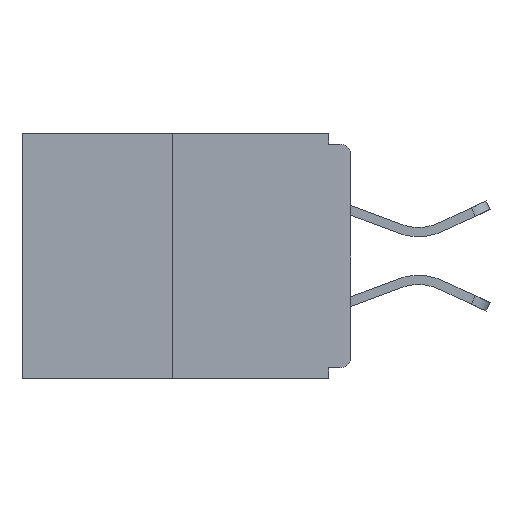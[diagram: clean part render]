
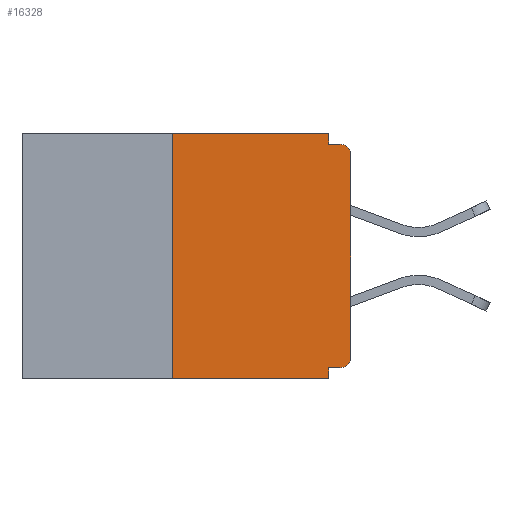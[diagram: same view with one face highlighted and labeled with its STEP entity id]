
A CAD part, left-side view. The second image highlights one B-rep face of the part: STEP entity #16328.
In plain terms, the highlighted planar face has unit normal (-1, 0, 0).
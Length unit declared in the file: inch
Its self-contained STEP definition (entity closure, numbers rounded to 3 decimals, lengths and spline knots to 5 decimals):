
#82 = VERTEX_POINT ( 'NONE', #6272 ) ;
#199 = CARTESIAN_POINT ( 'NONE',  ( 0., 0., -0.328 ) ) ;
#245 = CARTESIAN_POINT ( 'NONE',  ( 0., 0., -0.015 ) ) ;
#478 = VERTEX_POINT ( 'NONE', #7703 ) ;
#950 = ORIENTED_EDGE ( 'NONE', *, *, #20727, .T. ) ;
#986 = FACE_OUTER_BOUND ( 'NONE', #14619, .T. ) ;
#1017 = EDGE_CURVE ( 'NONE', #19914, #82, #13532, .T. ) ;
#1973 = CARTESIAN_POINT ( 'NONE',  ( 0., 0.031, 0. ) ) ;
#2096 = EDGE_CURVE ( 'NONE', #478, #8145, #9523, .T. ) ;
#2396 = CARTESIAN_POINT ( 'NONE',  ( 0., 0., 0. ) ) ;
#2826 = CARTESIAN_POINT ( 'NONE',  ( 0., 0.46, 0. ) ) ;
#3146 = VERTEX_POINT ( 'NONE', #3732 ) ;
#3207 = VECTOR ( 'NONE', #7239, 39.37008 ) ;
#3417 = VERTEX_POINT ( 'NONE', #3464 ) ;
#3464 = CARTESIAN_POINT ( 'NONE',  ( 0., 0.015, -0.328 ) ) ;
#3565 = LINE ( 'NONE', #245, #15094 ) ;
#3603 = VECTOR ( 'NONE', #21487, 39.37008 ) ;
#3732 = CARTESIAN_POINT ( 'NONE',  ( 0., 0.25, -0.343 ) ) ;
#4005 = VECTOR ( 'NONE', #13349, 39.37008 ) ;
#4217 = DIRECTION ( 'NONE',  ( 0., 0., -1. ) ) ;
#4445 = CARTESIAN_POINT ( 'NONE',  ( 0., 0.46, 0. ) ) ;
#4777 = VERTEX_POINT ( 'NONE', #11687 ) ;
#4943 = EDGE_CURVE ( 'NONE', #3417, #478, #10783, .T. ) ;
#5221 = ORIENTED_EDGE ( 'NONE', *, *, #20174, .T. ) ;
#5307 = CARTESIAN_POINT ( 'NONE',  ( 0., 0.25, 0. ) ) ;
#5667 = DIRECTION ( 'NONE',  ( 0., 0., -1. ) ) ;
#6024 = CIRCLE ( 'NONE', #18871, 0.015 ) ;
#6272 = CARTESIAN_POINT ( 'NONE',  ( 0., 0.031, -0.015 ) ) ;
#6292 = CARTESIAN_POINT ( 'NONE',  ( 0., 0.031, -0.343 ) ) ;
#6372 = EDGE_CURVE ( 'NONE', #3146, #19278, #20629, .T. ) ;
#6813 = EDGE_CURVE ( 'NONE', #3146, #8145, #17569, .T. ) ;
#6817 = CARTESIAN_POINT ( 'NONE',  ( 0., 0.25, 0. ) ) ;
#6891 = DIRECTION ( 'NONE',  ( 0., 0., 1. ) ) ;
#7239 = DIRECTION ( 'NONE',  ( 0., 0., 1. ) ) ;
#7465 = AXIS2_PLACEMENT_3D ( 'NONE', #8396, #17013, #11736 ) ;
#7703 = CARTESIAN_POINT ( 'NONE',  ( 0., 0.031, -0.328 ) ) ;
#8145 = VERTEX_POINT ( 'NONE', #12028 ) ;
#8396 = CARTESIAN_POINT ( 'NONE',  ( 0., 0.015, -0.03 ) ) ;
#8596 = DIRECTION ( 'NONE',  ( -1., 0., 0. ) ) ;
#8708 = CARTESIAN_POINT ( 'NONE',  ( 0., 0., -0.313 ) ) ;
#9095 = ORIENTED_EDGE ( 'NONE', *, *, #11487, .F. ) ;
#9523 = LINE ( 'NONE', #6292, #3603 ) ;
#10064 = VERTEX_POINT ( 'NONE', #8708 ) ;
#10783 = LINE ( 'NONE', #199, #12243 ) ;
#11331 = ORIENTED_EDGE ( 'NONE', *, *, #6813, .T. ) ;
#11487 = EDGE_CURVE ( 'NONE', #82, #12473, #3565, .T. ) ;
#11687 = CARTESIAN_POINT ( 'NONE',  ( 0., 0., -0.03 ) ) ;
#11736 = DIRECTION ( 'NONE',  ( 0., 0., -1. ) ) ;
#11744 = CARTESIAN_POINT ( 'NONE',  ( 0., 0.031, 0. ) ) ;
#12028 = CARTESIAN_POINT ( 'NONE',  ( 0., 0.031, -0.343 ) ) ;
#12156 = CARTESIAN_POINT ( 'NONE',  ( 0., 0.015, -0.313 ) ) ;
#12243 = VECTOR ( 'NONE', #15952, 39.37008 ) ;
#12285 = ORIENTED_EDGE ( 'NONE', *, *, #1017, .F. ) ;
#12473 = VERTEX_POINT ( 'NONE', #17759 ) ;
#12476 = ORIENTED_EDGE ( 'NONE', *, *, #2096, .F. ) ;
#12724 = PLANE ( 'NONE',  #20740 ) ;
#13349 = DIRECTION ( 'NONE',  ( 0., -1., 0. ) ) ;
#13532 = LINE ( 'NONE', #11744, #21991 ) ;
#13847 = ORIENTED_EDGE ( 'NONE', *, *, #15674, .T. ) ;
#14095 = CARTESIAN_POINT ( 'NONE',  ( 0., 0.46, -0.343 ) ) ;
#14318 = DIRECTION ( 'NONE',  ( 0., -1., 0. ) ) ;
#14619 = EDGE_LOOP ( 'NONE', ( #20937, #19117, #11331, #12476, #20571, #950, #13847, #5221, #9095, #12285 ) ) ;
#15094 = VECTOR ( 'NONE', #17110, 39.37008 ) ;
#15614 = LINE ( 'NONE', #2396, #3207 ) ;
#15674 = EDGE_CURVE ( 'NONE', #10064, #4777, #15614, .T. ) ;
#15817 = VECTOR ( 'NONE', #14318, 39.37008 ) ;
#15952 = DIRECTION ( 'NONE',  ( 0., 1., 0. ) ) ;
#16328 = ADVANCED_FACE ( 'NONE', ( #986 ), #12724, .F. ) ;
#16753 = CIRCLE ( 'NONE', #7465, 0.015 ) ;
#17013 = DIRECTION ( 'NONE',  ( -1., 0., 0. ) ) ;
#17110 = DIRECTION ( 'NONE',  ( 0., -1., 0. ) ) ;
#17569 = LINE ( 'NONE', #14095, #15817 ) ;
#17601 = EDGE_CURVE ( 'NONE', #19278, #19914, #18400, .T. ) ;
#17759 = CARTESIAN_POINT ( 'NONE',  ( 0., 0.015, -0.015 ) ) ;
#18098 = DIRECTION ( 'NONE',  ( 1., 0., 0. ) ) ;
#18400 = LINE ( 'NONE', #2826, #4005 ) ;
#18871 = AXIS2_PLACEMENT_3D ( 'NONE', #12156, #8596, #5667 ) ;
#19117 = ORIENTED_EDGE ( 'NONE', *, *, #6372, .F. ) ;
#19278 = VERTEX_POINT ( 'NONE', #6817 ) ;
#19914 = VERTEX_POINT ( 'NONE', #1973 ) ;
#20174 = EDGE_CURVE ( 'NONE', #4777, #12473, #16753, .T. ) ;
#20343 = DIRECTION ( 'NONE',  ( 0., 0., -1. ) ) ;
#20571 = ORIENTED_EDGE ( 'NONE', *, *, #4943, .F. ) ;
#20629 = LINE ( 'NONE', #5307, #21141 ) ;
#20727 = EDGE_CURVE ( 'NONE', #3417, #10064, #6024, .T. ) ;
#20740 = AXIS2_PLACEMENT_3D ( 'NONE', #4445, #18098, #4217 ) ;
#20937 = ORIENTED_EDGE ( 'NONE', *, *, #17601, .F. ) ;
#21141 = VECTOR ( 'NONE', #6891, 39.37008 ) ;
#21487 = DIRECTION ( 'NONE',  ( 0., 0., -1. ) ) ;
#21991 = VECTOR ( 'NONE', #20343, 39.37008 ) ;
